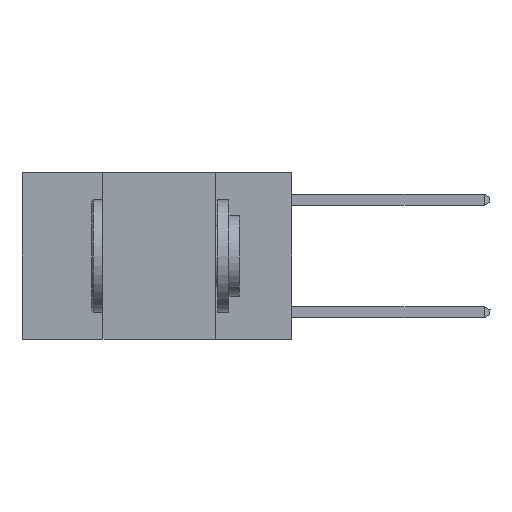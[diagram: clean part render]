
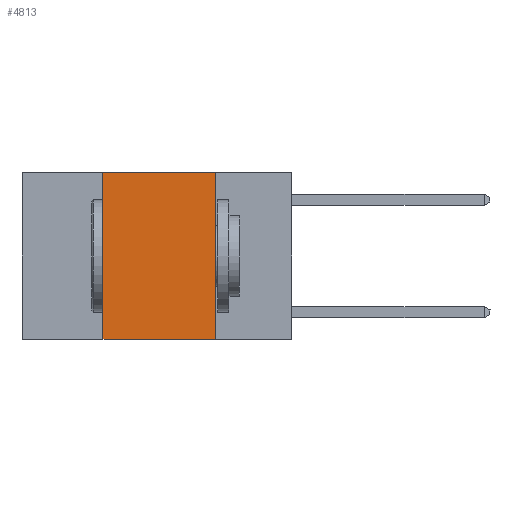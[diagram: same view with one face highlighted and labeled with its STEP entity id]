
A CAD part, left-side view. The second image highlights one B-rep face of the part: STEP entity #4813.
In plain terms, the highlighted planar face has unit normal (-1, 0, 0).
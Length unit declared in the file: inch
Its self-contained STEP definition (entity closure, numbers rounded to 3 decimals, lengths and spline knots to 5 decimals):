
#149 = CARTESIAN_POINT ( 'NONE',  ( 0., 0.6, 0. ) ) ;
#223 = VECTOR ( 'NONE', #4521, 39.37008 ) ;
#366 = EDGE_CURVE ( 'NONE', #3548, #1092, #7169, .T. ) ;
#485 = FACE_OUTER_BOUND ( 'NONE', #9223, .T. ) ;
#878 = EDGE_CURVE ( 'NONE', #10020, #3037, #7159, .T. ) ;
#1011 = DIRECTION ( 'NONE',  ( 0., 0., -1. ) ) ;
#1092 = VERTEX_POINT ( 'NONE', #3423 ) ;
#1221 = ORIENTED_EDGE ( 'NONE', *, *, #6495, .F. ) ;
#2042 = DIRECTION ( 'NONE',  ( 0., -1., 0. ) ) ;
#2125 = CARTESIAN_POINT ( 'NONE',  ( 0., 0.6, 0. ) ) ;
#2300 = LINE ( 'NONE', #9368, #223 ) ;
#2661 = VECTOR ( 'NONE', #2042, 39.37008 ) ;
#2724 = AXIS2_PLACEMENT_3D ( 'NONE', #149, #6238, #1011 ) ;
#3037 = VERTEX_POINT ( 'NONE', #10405 ) ;
#3423 = CARTESIAN_POINT ( 'NONE',  ( 0., 0.17, -0.37 ) ) ;
#3506 = EDGE_CURVE ( 'NONE', #3548, #10020, #8144, .T. ) ;
#3548 = VERTEX_POINT ( 'NONE', #6142 ) ;
#4436 = DIRECTION ( 'NONE',  ( 0., 0., 1. ) ) ;
#4521 = DIRECTION ( 'NONE',  ( 0., 0., -1. ) ) ;
#4713 = ORIENTED_EDGE ( 'NONE', *, *, #366, .T. ) ;
#4813 = ADVANCED_FACE ( 'NONE', ( #485 ), #10273, .F. ) ;
#6111 = CARTESIAN_POINT ( 'NONE',  ( 0., 0.42, 0. ) ) ;
#6142 = CARTESIAN_POINT ( 'NONE',  ( 0., 0.42, -0.37 ) ) ;
#6238 = DIRECTION ( 'NONE',  ( 1., 0., 0. ) ) ;
#6495 = EDGE_CURVE ( 'NONE', #3037, #1092, #2300, .T. ) ;
#6646 = ORIENTED_EDGE ( 'NONE', *, *, #878, .F. ) ;
#6793 = CARTESIAN_POINT ( 'NONE',  ( 0., 0.42, 0. ) ) ;
#7159 = LINE ( 'NONE', #2125, #2661 ) ;
#7169 = LINE ( 'NONE', #10557, #7429 ) ;
#7429 = VECTOR ( 'NONE', #8599, 39.37008 ) ;
#8144 = LINE ( 'NONE', #6111, #10288 ) ;
#8599 = DIRECTION ( 'NONE',  ( 0., -1., 0. ) ) ;
#8795 = ORIENTED_EDGE ( 'NONE', *, *, #3506, .F. ) ;
#9223 = EDGE_LOOP ( 'NONE', ( #1221, #6646, #8795, #4713 ) ) ;
#9368 = CARTESIAN_POINT ( 'NONE',  ( 0., 0.17, 0. ) ) ;
#10020 = VERTEX_POINT ( 'NONE', #6793 ) ;
#10273 = PLANE ( 'NONE',  #2724 ) ;
#10288 = VECTOR ( 'NONE', #4436, 39.37008 ) ;
#10405 = CARTESIAN_POINT ( 'NONE',  ( 0., 0.17, 0. ) ) ;
#10557 = CARTESIAN_POINT ( 'NONE',  ( 0., 0.6, -0.37 ) ) ;
